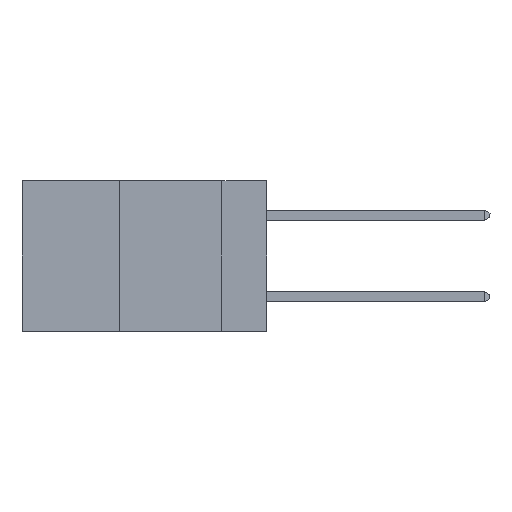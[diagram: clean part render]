
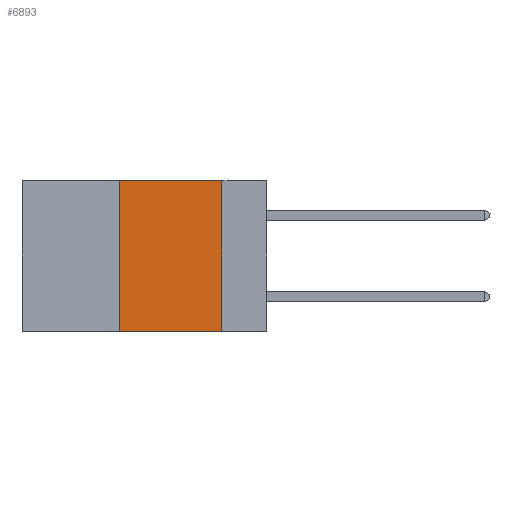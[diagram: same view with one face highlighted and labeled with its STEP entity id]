
A CAD part, left-side view. The second image highlights one B-rep face of the part: STEP entity #6893.
In plain terms, the highlighted planar face has unit normal (-1, 0, 0).
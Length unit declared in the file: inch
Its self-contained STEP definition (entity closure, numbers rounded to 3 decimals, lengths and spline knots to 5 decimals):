
#592 = VECTOR ( 'NONE', #6959, 39.37008 ) ;
#744 = VERTEX_POINT ( 'NONE', #3475 ) ;
#1025 = LINE ( 'NONE', #1181, #8086 ) ;
#1084 = DIRECTION ( 'NONE',  ( 0., 0., -1. ) ) ;
#1181 = CARTESIAN_POINT ( 'NONE',  ( 0., 0.11, 0. ) ) ;
#1841 = VECTOR ( 'NONE', #3864, 39.37008 ) ;
#2110 = CARTESIAN_POINT ( 'NONE',  ( 0., 0.36, 0. ) ) ;
#2213 = CARTESIAN_POINT ( 'NONE',  ( 0., 0.11, -0.37 ) ) ;
#2283 = CARTESIAN_POINT ( 'NONE',  ( 0., 0.6, -0.37 ) ) ;
#2736 = FACE_OUTER_BOUND ( 'NONE', #8795, .T. ) ;
#2958 = EDGE_CURVE ( 'NONE', #10666, #3710, #7198, .T. ) ;
#3475 = CARTESIAN_POINT ( 'NONE',  ( 0., 0.11, 0. ) ) ;
#3668 = ORIENTED_EDGE ( 'NONE', *, *, #6011, .F. ) ;
#3710 = VERTEX_POINT ( 'NONE', #7573 ) ;
#3864 = DIRECTION ( 'NONE',  ( 0., 0., 1. ) ) ;
#4646 = LINE ( 'NONE', #2283, #9654 ) ;
#5058 = ORIENTED_EDGE ( 'NONE', *, *, #2958, .F. ) ;
#6000 = ORIENTED_EDGE ( 'NONE', *, *, #9059, .F. ) ;
#6011 = EDGE_CURVE ( 'NONE', #744, #9838, #1025, .T. ) ;
#6076 = PLANE ( 'NONE',  #6344 ) ;
#6230 = CARTESIAN_POINT ( 'NONE',  ( 0., 0.6, 0. ) ) ;
#6344 = AXIS2_PLACEMENT_3D ( 'NONE', #6230, #7874, #1084 ) ;
#6893 = ADVANCED_FACE ( 'NONE', ( #2736 ), #6076, .F. ) ;
#6959 = DIRECTION ( 'NONE',  ( 0., -1., 0. ) ) ;
#6991 = EDGE_CURVE ( 'NONE', #10666, #9838, #4646, .T. ) ;
#7198 = LINE ( 'NONE', #2110, #1841 ) ;
#7573 = CARTESIAN_POINT ( 'NONE',  ( 0., 0.36, 0. ) ) ;
#7680 = CARTESIAN_POINT ( 'NONE',  ( 0., 0.36, -0.37 ) ) ;
#7783 = CARTESIAN_POINT ( 'NONE',  ( 0., 0.6, 0. ) ) ;
#7874 = DIRECTION ( 'NONE',  ( 1., 0., 0. ) ) ;
#8085 = ORIENTED_EDGE ( 'NONE', *, *, #6991, .T. ) ;
#8086 = VECTOR ( 'NONE', #9272, 39.37008 ) ;
#8593 = LINE ( 'NONE', #7783, #592 ) ;
#8795 = EDGE_LOOP ( 'NONE', ( #3668, #6000, #5058, #8085 ) ) ;
#9059 = EDGE_CURVE ( 'NONE', #3710, #744, #8593, .T. ) ;
#9272 = DIRECTION ( 'NONE',  ( 0., 0., -1. ) ) ;
#9599 = DIRECTION ( 'NONE',  ( 0., -1., 0. ) ) ;
#9654 = VECTOR ( 'NONE', #9599, 39.37008 ) ;
#9838 = VERTEX_POINT ( 'NONE', #2213 ) ;
#10666 = VERTEX_POINT ( 'NONE', #7680 ) ;
